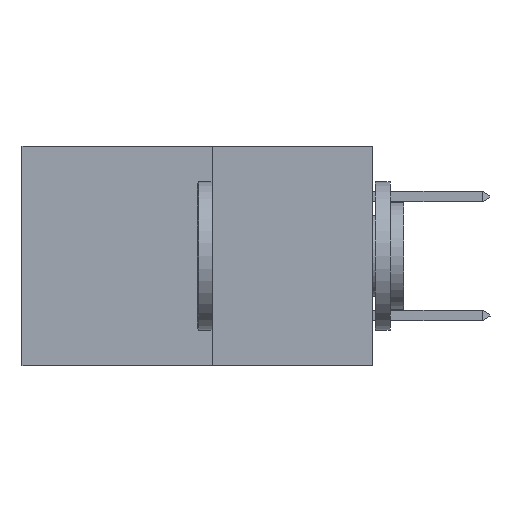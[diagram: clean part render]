
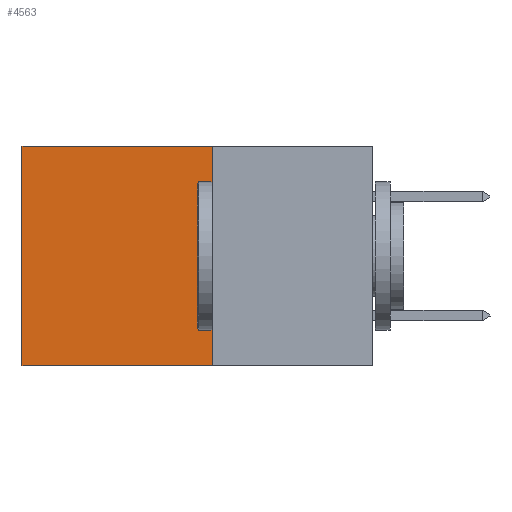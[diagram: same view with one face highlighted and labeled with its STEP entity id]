
A CAD part, left-side view. The second image highlights one B-rep face of the part: STEP entity #4563.
In plain terms, the highlighted planar face has unit normal (-1, 0, 0).
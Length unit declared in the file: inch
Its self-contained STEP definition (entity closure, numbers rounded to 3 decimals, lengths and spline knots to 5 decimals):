
#132 = VECTOR ( 'NONE', #7953, 39.37008 ) ;
#1663 = EDGE_CURVE ( 'NONE', #4279, #5604, #7742, .T. ) ;
#2354 = CARTESIAN_POINT ( 'NONE',  ( 0.277, 0.59, 0. ) ) ;
#2420 = AXIS2_PLACEMENT_3D ( 'NONE', #7907, #7793, #7780 ) ;
#2703 = VECTOR ( 'NONE', #5396, 39.37008 ) ;
#4279 = VERTEX_POINT ( 'NONE', #2354 ) ;
#4401 = EDGE_LOOP ( 'NONE', ( #8051, #6112, #10093, #10559 ) ) ;
#4563 = ADVANCED_FACE ( 'NONE', ( #9733 ), #7794, .F. ) ;
#4783 = LINE ( 'NONE', #6251, #2703 ) ;
#5247 = DIRECTION ( 'NONE',  ( 0., 1., 0. ) ) ;
#5396 = DIRECTION ( 'NONE',  ( 0., 1., 0. ) ) ;
#5517 = VECTOR ( 'NONE', #6488, 39.37008 ) ;
#5574 = VERTEX_POINT ( 'NONE', #7515 ) ;
#5604 = VERTEX_POINT ( 'NONE', #10607 ) ;
#5904 = VECTOR ( 'NONE', #5247, 39.37008 ) ;
#6112 = ORIENTED_EDGE ( 'NONE', *, *, #6802, .F. ) ;
#6251 = CARTESIAN_POINT ( 'NONE',  ( 0.277, 0.27, -0.37 ) ) ;
#6488 = DIRECTION ( 'NONE',  ( 0., 0., -1. ) ) ;
#6656 = EDGE_CURVE ( 'NONE', #5574, #4279, #10363, .T. ) ;
#6802 = EDGE_CURVE ( 'NONE', #7626, #5604, #4783, .T. ) ;
#7120 = CARTESIAN_POINT ( 'NONE',  ( 0.277, 0.27, -0.37 ) ) ;
#7515 = CARTESIAN_POINT ( 'NONE',  ( 0.277, 0.27, 0. ) ) ;
#7626 = VERTEX_POINT ( 'NONE', #9486 ) ;
#7742 = LINE ( 'NONE', #9279, #5517 ) ;
#7780 = DIRECTION ( 'NONE',  ( 0., 0., -1. ) ) ;
#7793 = DIRECTION ( 'NONE',  ( 1., 0., 0. ) ) ;
#7794 = PLANE ( 'NONE',  #2420 ) ;
#7907 = CARTESIAN_POINT ( 'NONE',  ( 0.277, 0.27, -0.37 ) ) ;
#7953 = DIRECTION ( 'NONE',  ( 0., 0., -1. ) ) ;
#8051 = ORIENTED_EDGE ( 'NONE', *, *, #1663, .T. ) ;
#9279 = CARTESIAN_POINT ( 'NONE',  ( 0.277, 0.59, -0.37 ) ) ;
#9287 = LINE ( 'NONE', #7120, #132 ) ;
#9486 = CARTESIAN_POINT ( 'NONE',  ( 0.277, 0.27, -0.37 ) ) ;
#9733 = FACE_OUTER_BOUND ( 'NONE', #4401, .T. ) ;
#10093 = ORIENTED_EDGE ( 'NONE', *, *, #10131, .F. ) ;
#10131 = EDGE_CURVE ( 'NONE', #5574, #7626, #9287, .T. ) ;
#10363 = LINE ( 'NONE', #10768, #5904 ) ;
#10559 = ORIENTED_EDGE ( 'NONE', *, *, #6656, .T. ) ;
#10607 = CARTESIAN_POINT ( 'NONE',  ( 0.277, 0.59, -0.37 ) ) ;
#10768 = CARTESIAN_POINT ( 'NONE',  ( 0.277, 0.27, 0. ) ) ;
